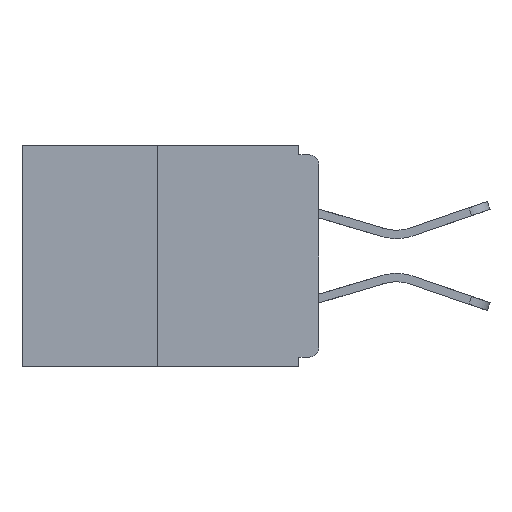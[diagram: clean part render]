
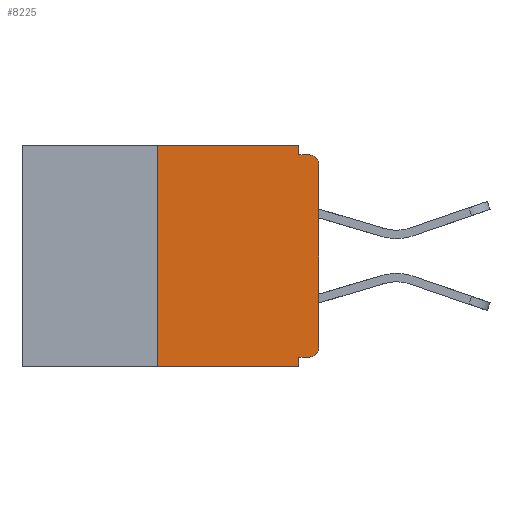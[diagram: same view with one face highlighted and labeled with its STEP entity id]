
A CAD part, left-side view. The second image highlights one B-rep face of the part: STEP entity #8225.
In plain terms, the highlighted planar face has unit normal (-1, 0, 0).
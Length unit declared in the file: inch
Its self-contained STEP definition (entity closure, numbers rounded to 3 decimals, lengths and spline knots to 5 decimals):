
#141 = VECTOR ( 'NONE', #5828, 39.37008 ) ;
#159 = DIRECTION ( 'NONE',  ( -1., 0., 0. ) ) ;
#272 = DIRECTION ( 'NONE',  ( 0., 0., 1. ) ) ;
#1054 = ORIENTED_EDGE ( 'NONE', *, *, #13772, .F. ) ;
#1463 = EDGE_CURVE ( 'NONE', #3181, #5148, #10912, .T. ) ;
#1487 = CARTESIAN_POINT ( 'NONE',  ( 0., 0.031, 0. ) ) ;
#1647 = ORIENTED_EDGE ( 'NONE', *, *, #3423, .F. ) ;
#1866 = DIRECTION ( 'NONE',  ( 0., -1., 0. ) ) ;
#1957 = CARTESIAN_POINT ( 'NONE',  ( 0., 0.015, -0.03 ) ) ;
#2062 = CARTESIAN_POINT ( 'NONE',  ( 0., 0.015, -0.015 ) ) ;
#2296 = ORIENTED_EDGE ( 'NONE', *, *, #13378, .T. ) ;
#2338 = AXIS2_PLACEMENT_3D ( 'NONE', #1957, #6431, #10007 ) ;
#2875 = ORIENTED_EDGE ( 'NONE', *, *, #14181, .T. ) ;
#3153 = CARTESIAN_POINT ( 'NONE',  ( 0., 0.031, -0.015 ) ) ;
#3181 = VERTEX_POINT ( 'NONE', #1487 ) ;
#3423 = EDGE_CURVE ( 'NONE', #5148, #6787, #8523, .T. ) ;
#3500 = ORIENTED_EDGE ( 'NONE', *, *, #13287, .T. ) ;
#3828 = VECTOR ( 'NONE', #1866, 39.37008 ) ;
#3998 = AXIS2_PLACEMENT_3D ( 'NONE', #12220, #8825, #4218 ) ;
#3999 = VECTOR ( 'NONE', #9024, 39.37008 ) ;
#4046 = LINE ( 'NONE', #10739, #7299 ) ;
#4218 = DIRECTION ( 'NONE',  ( 0., 0., -1. ) ) ;
#4261 = ORIENTED_EDGE ( 'NONE', *, *, #1463, .F. ) ;
#4407 = CARTESIAN_POINT ( 'NONE',  ( 0., 0.031, -0.343 ) ) ;
#4411 = ORIENTED_EDGE ( 'NONE', *, *, #9110, .F. ) ;
#4706 = CARTESIAN_POINT ( 'NONE',  ( 0., 0.031, -0.328 ) ) ;
#4813 = DIRECTION ( 'NONE',  ( 0., 0., -1. ) ) ;
#4839 = DIRECTION ( 'NONE',  ( 0., 0., -1. ) ) ;
#4932 = EDGE_CURVE ( 'NONE', #14746, #11744, #6349, .T. ) ;
#4983 = CARTESIAN_POINT ( 'NONE',  ( 0., 0., -0.03 ) ) ;
#5148 = VERTEX_POINT ( 'NONE', #3153 ) ;
#5668 = CARTESIAN_POINT ( 'NONE',  ( 0., 0., -0.328 ) ) ;
#5828 = DIRECTION ( 'NONE',  ( 0., 0., -1. ) ) ;
#6304 = CARTESIAN_POINT ( 'NONE',  ( 0., 0.46, -0.343 ) ) ;
#6349 = LINE ( 'NONE', #5668, #8880 ) ;
#6431 = DIRECTION ( 'NONE',  ( -1., 0., 0. ) ) ;
#6524 = CARTESIAN_POINT ( 'NONE',  ( 0., 0., -0.015 ) ) ;
#6559 = CARTESIAN_POINT ( 'NONE',  ( 0., 0., -0.313 ) ) ;
#6566 = VERTEX_POINT ( 'NONE', #7080 ) ;
#6787 = VERTEX_POINT ( 'NONE', #2062 ) ;
#7024 = DIRECTION ( 'NONE',  ( 0., -1., 0. ) ) ;
#7080 = CARTESIAN_POINT ( 'NONE',  ( 0., 0.031, -0.343 ) ) ;
#7299 = VECTOR ( 'NONE', #13046, 39.37008 ) ;
#7360 = VERTEX_POINT ( 'NONE', #4983 ) ;
#7581 = VECTOR ( 'NONE', #4813, 39.37008 ) ;
#8197 = EDGE_LOOP ( 'NONE', ( #4411, #1054, #2875, #10443, #12930, #3500, #8299, #2296, #1647, #4261 ) ) ;
#8225 = ADVANCED_FACE ( 'NONE', ( #12731 ), #10072, .F. ) ;
#8249 = CARTESIAN_POINT ( 'NONE',  ( 0., 0.25, 0. ) ) ;
#8299 = ORIENTED_EDGE ( 'NONE', *, *, #12051, .T. ) ;
#8523 = LINE ( 'NONE', #6524, #3828 ) ;
#8825 = DIRECTION ( 'NONE',  ( 1., 0., 0. ) ) ;
#8880 = VECTOR ( 'NONE', #10350, 39.37008 ) ;
#9024 = DIRECTION ( 'NONE',  ( 0., 0., 1. ) ) ;
#9110 = EDGE_CURVE ( 'NONE', #11386, #3181, #4046, .T. ) ;
#9253 = CARTESIAN_POINT ( 'NONE',  ( 0., 0.031, 0. ) ) ;
#9371 = VERTEX_POINT ( 'NONE', #6559 ) ;
#9378 = CIRCLE ( 'NONE', #2338, 0.015 ) ;
#10007 = DIRECTION ( 'NONE',  ( 0., 0., -1. ) ) ;
#10072 = PLANE ( 'NONE',  #3998 ) ;
#10277 = CIRCLE ( 'NONE', #13408, 0.015 ) ;
#10340 = EDGE_CURVE ( 'NONE', #11744, #6566, #11052, .T. ) ;
#10350 = DIRECTION ( 'NONE',  ( 0., 1., 0. ) ) ;
#10443 = ORIENTED_EDGE ( 'NONE', *, *, #10340, .F. ) ;
#10739 = CARTESIAN_POINT ( 'NONE',  ( 0., 0.46, 0. ) ) ;
#10823 = VECTOR ( 'NONE', #272, 39.37008 ) ;
#10912 = LINE ( 'NONE', #9253, #141 ) ;
#10915 = VERTEX_POINT ( 'NONE', #14481 ) ;
#11052 = LINE ( 'NONE', #4407, #7581 ) ;
#11386 = VERTEX_POINT ( 'NONE', #8249 ) ;
#11711 = CARTESIAN_POINT ( 'NONE',  ( 0., 0.25, 0. ) ) ;
#11744 = VERTEX_POINT ( 'NONE', #4706 ) ;
#11888 = LINE ( 'NONE', #11711, #10823 ) ;
#12051 = EDGE_CURVE ( 'NONE', #9371, #7360, #12278, .T. ) ;
#12209 = VECTOR ( 'NONE', #7024, 39.37008 ) ;
#12220 = CARTESIAN_POINT ( 'NONE',  ( 0., 0.46, 0. ) ) ;
#12278 = LINE ( 'NONE', #13525, #3999 ) ;
#12467 = CARTESIAN_POINT ( 'NONE',  ( 0., 0.015, -0.328 ) ) ;
#12731 = FACE_OUTER_BOUND ( 'NONE', #8197, .T. ) ;
#12930 = ORIENTED_EDGE ( 'NONE', *, *, #4932, .F. ) ;
#13046 = DIRECTION ( 'NONE',  ( 0., -1., 0. ) ) ;
#13287 = EDGE_CURVE ( 'NONE', #14746, #9371, #10277, .T. ) ;
#13304 = LINE ( 'NONE', #6304, #12209 ) ;
#13378 = EDGE_CURVE ( 'NONE', #7360, #6787, #9378, .T. ) ;
#13408 = AXIS2_PLACEMENT_3D ( 'NONE', #13873, #159, #4839 ) ;
#13525 = CARTESIAN_POINT ( 'NONE',  ( 0., 0., 0. ) ) ;
#13772 = EDGE_CURVE ( 'NONE', #10915, #11386, #11888, .T. ) ;
#13873 = CARTESIAN_POINT ( 'NONE',  ( 0., 0.015, -0.313 ) ) ;
#14181 = EDGE_CURVE ( 'NONE', #10915, #6566, #13304, .T. ) ;
#14481 = CARTESIAN_POINT ( 'NONE',  ( 0., 0.25, -0.343 ) ) ;
#14746 = VERTEX_POINT ( 'NONE', #12467 ) ;
